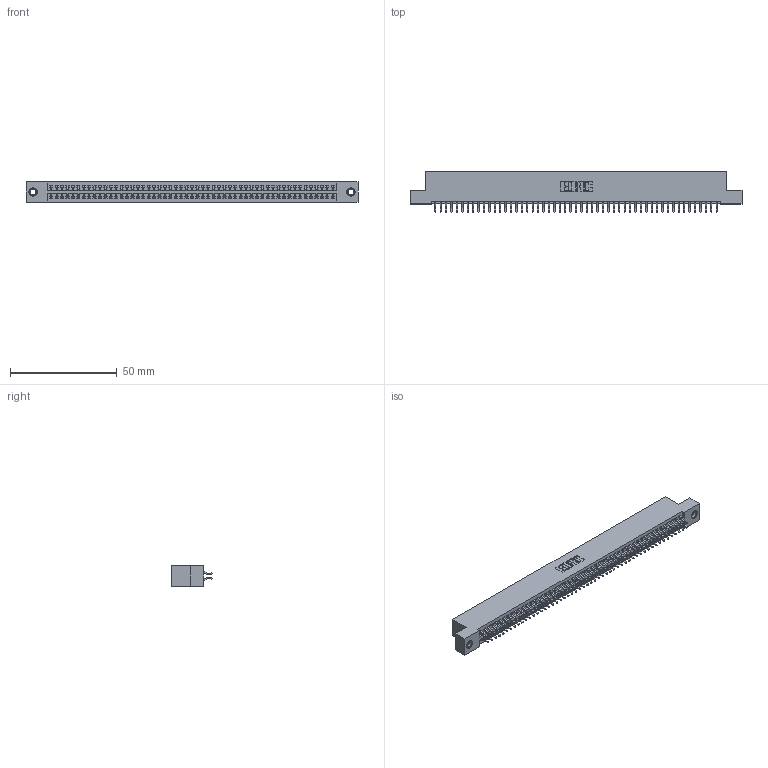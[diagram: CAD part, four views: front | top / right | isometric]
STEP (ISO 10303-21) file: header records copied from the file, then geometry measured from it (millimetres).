
FILE_DESCRIPTION (( 'STEP AP203' ), '1' );
FILE_NAME ('345-106-556-207.STEP', '2019-11-03T17:17:29', ( '' ), ( '' ), 'SwSTEP 2.0', 'SolidWorks 2016', '' );
FILE_SCHEMA (( 'CONFIG_CONTROL_DESIGN' ));
Length unit declared in the file: inch
Products named in the file (4): 345 Part_Flush Mounting Lugs - 0.156 Dia-TI; 345-250-001_345-250-005-103; 345-106-556-207; 345-292-001_556 Tail
Assembly tree (109 placements, depth 2):
  345-106-556-207
    345 Part_Flush Mounting Lugs - 0.156 Dia-TI
    345-292-001_556 Tail  x106
    345-250-001_345-250-005-103  x2
Bounding box: 155.83 x 19.24 x 9.4 mm (x, y, z)
Volume: 15221.8 mm3; surface area: 22648.5 mm2
Topology: 109 solids, 109 shells, 6122 faces, 18179 edges, 11970 vertices
Faces by surface type: plane 4034, cylinder 2072, cone 12, torus 4
Entity records: 41510 total; most frequent: CARTESIAN_POINT 6943, ORIENTED_EDGE 6858, DIRECTION 6123, EDGE_CURVE 3429, LINE 3057, VECTOR 3057, VERTEX_POINT 2280, AXIS2_PLACEMENT_3D 1533
